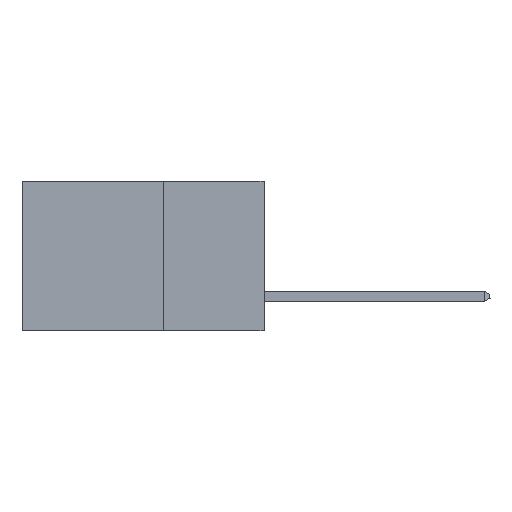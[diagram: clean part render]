
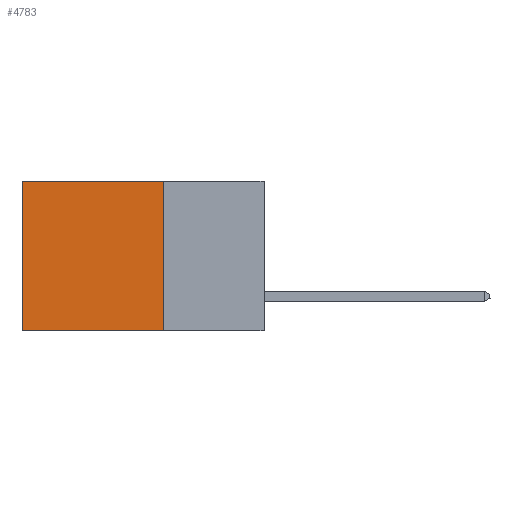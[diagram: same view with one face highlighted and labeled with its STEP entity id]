
A CAD part, left-side view. The second image highlights one B-rep face of the part: STEP entity #4783.
In plain terms, the highlighted planar face has unit normal (-1, 0, 0).
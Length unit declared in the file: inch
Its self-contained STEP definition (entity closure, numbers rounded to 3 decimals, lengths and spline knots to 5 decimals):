
#511 = VECTOR ( 'NONE', #13975, 39.37008 ) ;
#764 = VECTOR ( 'NONE', #13216, 39.37008 ) ;
#1391 = VECTOR ( 'NONE', #8663, 39.37008 ) ;
#1515 = CARTESIAN_POINT ( 'NONE',  ( 0.2615, 0.25, 0. ) ) ;
#1527 = CARTESIAN_POINT ( 'NONE',  ( 0.2615, 0.25, -0.37 ) ) ;
#1966 = EDGE_CURVE ( 'NONE', #7961, #9075, #13589, .T. ) ;
#3574 = ORIENTED_EDGE ( 'NONE', *, *, #6676, .T. ) ;
#3617 = ORIENTED_EDGE ( 'NONE', *, *, #8403, .F. ) ;
#3655 = CARTESIAN_POINT ( 'NONE',  ( 0.2615, 0.25, -0.37 ) ) ;
#3798 = CARTESIAN_POINT ( 'NONE',  ( 0.2615, 0.6, -0.37 ) ) ;
#3835 = DIRECTION ( 'NONE',  ( 0., 0., -1. ) ) ;
#3944 = PLANE ( 'NONE',  #10288 ) ;
#4474 = ORIENTED_EDGE ( 'NONE', *, *, #11817, .F. ) ;
#4713 = CARTESIAN_POINT ( 'NONE',  ( 0.2615, 0.25, 0. ) ) ;
#4783 = ADVANCED_FACE ( 'NONE', ( #7124 ), #3944, .F. ) ;
#5759 = CARTESIAN_POINT ( 'NONE',  ( 0.2615, 0.6, 0. ) ) ;
#6676 = EDGE_CURVE ( 'NONE', #9699, #7961, #11550, .T. ) ;
#7124 = FACE_OUTER_BOUND ( 'NONE', #9134, .T. ) ;
#7535 = LINE ( 'NONE', #9922, #764 ) ;
#7961 = VERTEX_POINT ( 'NONE', #5759 ) ;
#8403 = EDGE_CURVE ( 'NONE', #9699, #10915, #13057, .T. ) ;
#8663 = DIRECTION ( 'NONE',  ( 0., 0., -1. ) ) ;
#9075 = VERTEX_POINT ( 'NONE', #3798 ) ;
#9134 = EDGE_LOOP ( 'NONE', ( #9915, #4474, #3617, #3574 ) ) ;
#9512 = DIRECTION ( 'NONE',  ( 1., 0., 0. ) ) ;
#9699 = VERTEX_POINT ( 'NONE', #4713 ) ;
#9915 = ORIENTED_EDGE ( 'NONE', *, *, #1966, .T. ) ;
#9922 = CARTESIAN_POINT ( 'NONE',  ( 0.2615, 0.25, -0.37 ) ) ;
#10288 = AXIS2_PLACEMENT_3D ( 'NONE', #1527, #9512, #3835 ) ;
#10915 = VERTEX_POINT ( 'NONE', #12100 ) ;
#11195 = VECTOR ( 'NONE', #11772, 39.37008 ) ;
#11550 = LINE ( 'NONE', #1515, #11195 ) ;
#11772 = DIRECTION ( 'NONE',  ( 0., 1., 0. ) ) ;
#11817 = EDGE_CURVE ( 'NONE', #10915, #9075, #7535, .T. ) ;
#12100 = CARTESIAN_POINT ( 'NONE',  ( 0.2615, 0.25, -0.37 ) ) ;
#13057 = LINE ( 'NONE', #3655, #511 ) ;
#13066 = CARTESIAN_POINT ( 'NONE',  ( 0.2615, 0.6, -0.37 ) ) ;
#13216 = DIRECTION ( 'NONE',  ( 0., 1., 0. ) ) ;
#13589 = LINE ( 'NONE', #13066, #1391 ) ;
#13975 = DIRECTION ( 'NONE',  ( 0., 0., -1. ) ) ;
